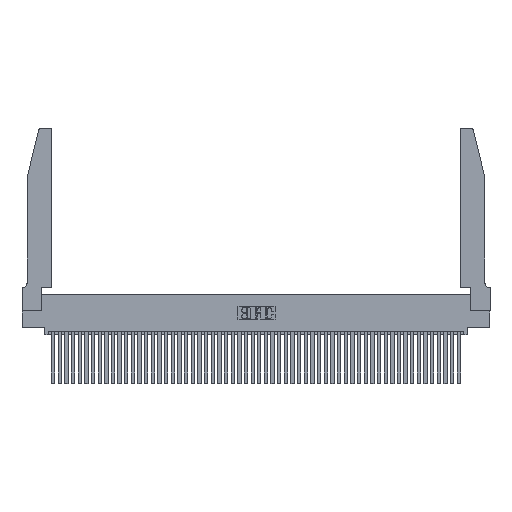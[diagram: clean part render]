
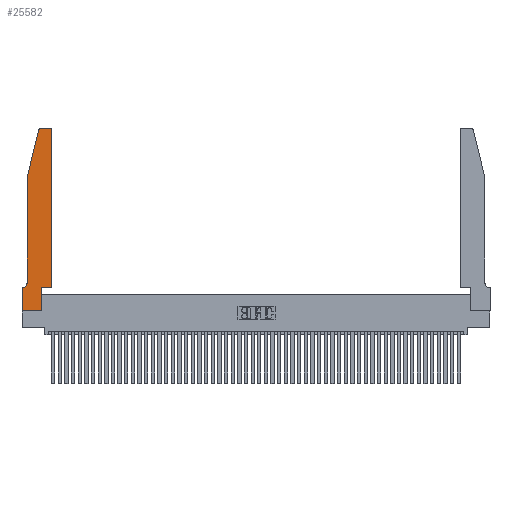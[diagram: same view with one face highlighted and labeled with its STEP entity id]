
A CAD part, top view. The second image highlights one B-rep face of the part: STEP entity #25582.
In plain terms, the highlighted planar face has unit normal (0, 0, 1).
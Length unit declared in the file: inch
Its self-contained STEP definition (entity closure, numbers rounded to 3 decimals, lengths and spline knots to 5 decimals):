
#427 = CIRCLE ( 'NONE', #6920, 0.03 ) ;
#616 = CARTESIAN_POINT ( 'NONE',  ( 0.2865, 0.35, 0.37 ) ) ;
#659 = VERTEX_POINT ( 'NONE', #616 ) ;
#1928 = CARTESIAN_POINT ( 'NONE',  ( 0.4205, 2.75, 0.37 ) ) ;
#2405 = DIRECTION ( 'NONE',  ( 0., 0., 1. ) ) ;
#2982 = CARTESIAN_POINT ( 'NONE',  ( 0.0755, 0.42, 0.37 ) ) ;
#3055 = VECTOR ( 'NONE', #40448, 39.37008 ) ;
#3073 = VERTEX_POINT ( 'NONE', #41588 ) ;
#3327 = VECTOR ( 'NONE', #46577, 39.37008 ) ;
#3356 = VECTOR ( 'NONE', #10413, 39.37008 ) ;
#4540 = EDGE_CURVE ( 'NONE', #40741, #11043, #29871, .T. ) ;
#5341 = ORIENTED_EDGE ( 'NONE', *, *, #27100, .T. ) ;
#6383 = CARTESIAN_POINT ( 'NONE',  ( 0.0755, 2., 0.37 ) ) ;
#6644 = CARTESIAN_POINT ( 'NONE',  ( 0.2865, 0., 0.37 ) ) ;
#6791 = DIRECTION ( 'NONE',  ( 0., 0., -1. ) ) ;
#6920 = AXIS2_PLACEMENT_3D ( 'NONE', #14072, #41304, #18016 ) ;
#7095 = ORIENTED_EDGE ( 'NONE', *, *, #48985, .T. ) ;
#7703 = CARTESIAN_POINT ( 'NONE',  ( 0.0755, 2., 0.37 ) ) ;
#8016 = DIRECTION ( 'NONE',  ( 0., 1., 0. ) ) ;
#8315 = CARTESIAN_POINT ( 'NONE',  ( 0.284, 2.75, 0.37 ) ) ;
#9075 = EDGE_CURVE ( 'NONE', #19518, #9358, #427, .T. ) ;
#9129 = EDGE_CURVE ( 'NONE', #33908, #40741, #50032, .T. ) ;
#9358 = VERTEX_POINT ( 'NONE', #1928 ) ;
#9804 = ORIENTED_EDGE ( 'NONE', *, *, #48739, .T. ) ;
#10413 = DIRECTION ( 'NONE',  ( 0., -1., 0. ) ) ;
#10490 = ORIENTED_EDGE ( 'NONE', *, *, #39355, .T. ) ;
#10801 = EDGE_LOOP ( 'NONE', ( #5341, #48375, #12926, #11106, #10490, #7095, #19543, #9804, #36021, #12560, #35034, #38047 ) ) ;
#11043 = VERTEX_POINT ( 'NONE', #31539 ) ;
#11106 = ORIENTED_EDGE ( 'NONE', *, *, #30775, .T. ) ;
#11754 = VERTEX_POINT ( 'NONE', #31991 ) ;
#11909 = CARTESIAN_POINT ( 'NONE',  ( 0.4505, 0.35, 0.37 ) ) ;
#12260 = AXIS2_PLACEMENT_3D ( 'NONE', #26052, #2405, #29965 ) ;
#12560 = ORIENTED_EDGE ( 'NONE', *, *, #26550, .T. ) ;
#12926 = ORIENTED_EDGE ( 'NONE', *, *, #4540, .T. ) ;
#13104 = EDGE_CURVE ( 'NONE', #39618, #3073, #39995, .T. ) ;
#13394 = CARTESIAN_POINT ( 'NONE',  ( 0., 0.35, 0.37 ) ) ;
#13570 = PLANE ( 'NONE',  #28455 ) ;
#14072 = CARTESIAN_POINT ( 'NONE',  ( 0.4205, 2.72, 0.37 ) ) ;
#15026 = LINE ( 'NONE', #24253, #44826 ) ;
#15200 = LINE ( 'NONE', #6383, #3356 ) ;
#16331 = VERTEX_POINT ( 'NONE', #2982 ) ;
#17096 = AXIS2_PLACEMENT_3D ( 'NONE', #30320, #6791, #34240 ) ;
#17136 = CARTESIAN_POINT ( 'NONE',  ( 0.2605, 2.75, 0.37 ) ) ;
#17518 = DIRECTION ( 'NONE',  ( 1., 0., 0. ) ) ;
#17572 = FACE_OUTER_BOUND ( 'NONE', #10801, .T. ) ;
#18016 = DIRECTION ( 'NONE',  ( 1., 0., 0. ) ) ;
#18272 = VECTOR ( 'NONE', #19629, 39.37008 ) ;
#18626 = DIRECTION ( 'NONE',  ( -1., 0., 0. ) ) ;
#19425 = CARTESIAN_POINT ( 'NONE',  ( 0.4505, 0.35, 0.37 ) ) ;
#19518 = VERTEX_POINT ( 'NONE', #41538 ) ;
#19543 = ORIENTED_EDGE ( 'NONE', *, *, #13104, .T. ) ;
#19629 = DIRECTION ( 'NONE',  ( -0.239, -0.971, 0. ) ) ;
#22229 = DIRECTION ( 'NONE',  ( 0., -1., 0. ) ) ;
#23059 = CIRCLE ( 'NONE', #17096, 0.07 ) ;
#23118 = LINE ( 'NONE', #19425, #3327 ) ;
#23547 = LINE ( 'NONE', #38046, #32725 ) ;
#24051 = LINE ( 'NONE', #17136, #3055 ) ;
#24253 = CARTESIAN_POINT ( 'NONE',  ( 0., 0., 0.37 ) ) ;
#25248 = EDGE_CURVE ( 'NONE', #11754, #19518, #23118, .T. ) ;
#25431 = LINE ( 'NONE', #11909, #46043 ) ;
#25582 = ADVANCED_FACE ( 'NONE', ( #17572 ), #13570, .T. ) ;
#26052 = CARTESIAN_POINT ( 'NONE',  ( 0.284, 2.72, 0.37 ) ) ;
#26550 = EDGE_CURVE ( 'NONE', #659, #11754, #25431, .T. ) ;
#26797 = CARTESIAN_POINT ( 'NONE',  ( 0.25487, 2.72718, 0.37 ) ) ;
#27100 = EDGE_CURVE ( 'NONE', #9358, #33908, #24051, .T. ) ;
#27606 = CARTESIAN_POINT ( 'NONE',  ( 0.2865, 0.35, 0.37 ) ) ;
#28182 = DIRECTION ( 'NONE',  ( 1., 0., 0. ) ) ;
#28455 = AXIS2_PLACEMENT_3D ( 'NONE', #13394, #40826, #17518 ) ;
#29512 = VERTEX_POINT ( 'NONE', #43434 ) ;
#29871 = LINE ( 'NONE', #7703, #18272 ) ;
#29965 = DIRECTION ( 'NONE',  ( 1., 0., 0. ) ) ;
#30101 = LINE ( 'NONE', #27606, #39186 ) ;
#30320 = CARTESIAN_POINT ( 'NONE',  ( 0.0055, 0.42, 0.37 ) ) ;
#30775 = EDGE_CURVE ( 'NONE', #11043, #16331, #15200, .T. ) ;
#31539 = CARTESIAN_POINT ( 'NONE',  ( 0.0755, 2., 0.37 ) ) ;
#31991 = CARTESIAN_POINT ( 'NONE',  ( 0.4505, 0.35, 0.37 ) ) ;
#32725 = VECTOR ( 'NONE', #18626, 39.37008 ) ;
#33908 = VERTEX_POINT ( 'NONE', #8315 ) ;
#34240 = DIRECTION ( 'NONE',  ( -1., 0., 0. ) ) ;
#35034 = ORIENTED_EDGE ( 'NONE', *, *, #25248, .T. ) ;
#36021 = ORIENTED_EDGE ( 'NONE', *, *, #40921, .T. ) ;
#37600 = VECTOR ( 'NONE', #22229, 39.37008 ) ;
#38046 = CARTESIAN_POINT ( 'NONE',  ( 0.0755, 0.35, 0.37 ) ) ;
#38047 = ORIENTED_EDGE ( 'NONE', *, *, #9075, .T. ) ;
#39186 = VECTOR ( 'NONE', #8016, 39.37008 ) ;
#39197 = DIRECTION ( 'NONE',  ( 1., 0., 0. ) ) ;
#39267 = CARTESIAN_POINT ( 'NONE',  ( 0., 0.35, 0.37 ) ) ;
#39355 = EDGE_CURVE ( 'NONE', #16331, #29512, #23059, .T. ) ;
#39618 = VERTEX_POINT ( 'NONE', #39267 ) ;
#39995 = LINE ( 'NONE', #41580, #37600 ) ;
#40448 = DIRECTION ( 'NONE',  ( -1., 0., 0. ) ) ;
#40741 = VERTEX_POINT ( 'NONE', #26797 ) ;
#40826 = DIRECTION ( 'NONE',  ( 0., 0., 1. ) ) ;
#40921 = EDGE_CURVE ( 'NONE', #49707, #659, #30101, .T. ) ;
#41304 = DIRECTION ( 'NONE',  ( 0., 0., 1. ) ) ;
#41538 = CARTESIAN_POINT ( 'NONE',  ( 0.4505, 2.72, 0.37 ) ) ;
#41580 = CARTESIAN_POINT ( 'NONE',  ( 0., 0., 0.37 ) ) ;
#41588 = CARTESIAN_POINT ( 'NONE',  ( 0., 0., 0.37 ) ) ;
#43434 = CARTESIAN_POINT ( 'NONE',  ( 0.0055, 0.35, 0.37 ) ) ;
#44826 = VECTOR ( 'NONE', #28182, 39.37008 ) ;
#46043 = VECTOR ( 'NONE', #39197, 39.37008 ) ;
#46577 = DIRECTION ( 'NONE',  ( 0., 1., 0. ) ) ;
#48375 = ORIENTED_EDGE ( 'NONE', *, *, #9129, .T. ) ;
#48739 = EDGE_CURVE ( 'NONE', #3073, #49707, #15026, .T. ) ;
#48985 = EDGE_CURVE ( 'NONE', #29512, #39618, #23547, .T. ) ;
#49707 = VERTEX_POINT ( 'NONE', #6644 ) ;
#50032 = CIRCLE ( 'NONE', #12260, 0.03 ) ;
